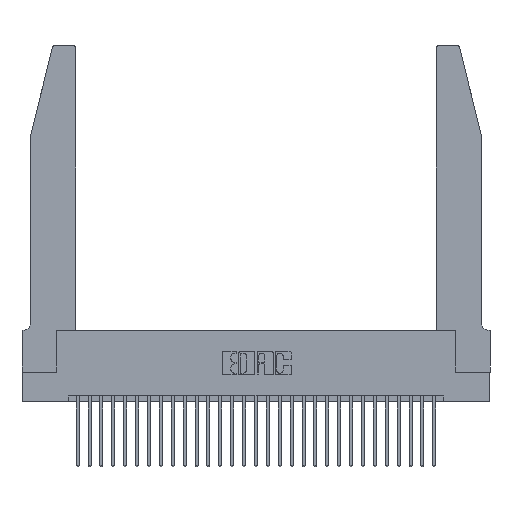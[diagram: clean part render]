
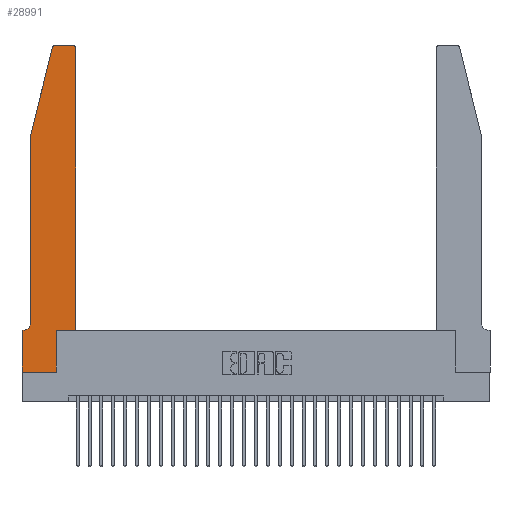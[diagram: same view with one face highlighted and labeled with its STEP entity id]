
A CAD part, top view. The second image highlights one B-rep face of the part: STEP entity #28991.
In plain terms, the highlighted planar face has unit normal (0, 0, 1).
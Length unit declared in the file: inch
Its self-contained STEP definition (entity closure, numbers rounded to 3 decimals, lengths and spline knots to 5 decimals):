
#165 = VECTOR ( 'NONE', #12756, 39.37008 ) ;
#220 = EDGE_CURVE ( 'NONE', #2170, #4722, #12702, .T. ) ;
#1205 = VECTOR ( 'NONE', #4119, 39.37008 ) ;
#1539 = ORIENTED_EDGE ( 'NONE', *, *, #20435, .T. ) ;
#1546 = LINE ( 'NONE', #21854, #14168 ) ;
#1667 = ORIENTED_EDGE ( 'NONE', *, *, #12171, .T. ) ;
#2170 = VERTEX_POINT ( 'NONE', #16006 ) ;
#2358 = CARTESIAN_POINT ( 'NONE',  ( 0.0055, 0.42, 0.37 ) ) ;
#3469 = EDGE_LOOP ( 'NONE', ( #22981, #5084, #25756, #27916, #11546, #19803, #18902, #1539, #1667, #20154, #10247, #19961 ) ) ;
#3696 = CARTESIAN_POINT ( 'NONE',  ( 0.4505, 0.35, 0.37 ) ) ;
#3702 = CARTESIAN_POINT ( 'NONE',  ( 0.4205, 2.72, 0.37 ) ) ;
#3861 = VERTEX_POINT ( 'NONE', #10319 ) ;
#4119 = DIRECTION ( 'NONE',  ( 0., -1., 0. ) ) ;
#4722 = VERTEX_POINT ( 'NONE', #16071 ) ;
#4742 = DIRECTION ( 'NONE',  ( -1., 0., 0. ) ) ;
#5084 = ORIENTED_EDGE ( 'NONE', *, *, #29666, .T. ) ;
#5510 = DIRECTION ( 'NONE',  ( -0.239, -0.971, 0. ) ) ;
#6071 = DIRECTION ( 'NONE',  ( 0., 1., 0. ) ) ;
#6081 = DIRECTION ( 'NONE',  ( 1., 0., 0. ) ) ;
#6169 = CARTESIAN_POINT ( 'NONE',  ( 0.25487, 2.72718, 0.37 ) ) ;
#6411 = VECTOR ( 'NONE', #6950, 39.37008 ) ;
#6533 = LINE ( 'NONE', #10378, #165 ) ;
#6630 = VECTOR ( 'NONE', #6666, 39.37008 ) ;
#6666 = DIRECTION ( 'NONE',  ( 0., -1., 0. ) ) ;
#6726 = EDGE_CURVE ( 'NONE', #9099, #27608, #6533, .T. ) ;
#6950 = DIRECTION ( 'NONE',  ( 1., 0., 0. ) ) ;
#7416 = EDGE_CURVE ( 'NONE', #28107, #9787, #12413, .T. ) ;
#7715 = DIRECTION ( 'NONE',  ( -1., 0., 0. ) ) ;
#7949 = DIRECTION ( 'NONE',  ( 1., 0., 0. ) ) ;
#8011 = CARTESIAN_POINT ( 'NONE',  ( 0.284, 2.72, 0.37 ) ) ;
#8129 = AXIS2_PLACEMENT_3D ( 'NONE', #3702, #20229, #6081 ) ;
#8808 = CARTESIAN_POINT ( 'NONE',  ( 0., 0., 0.37 ) ) ;
#8992 = AXIS2_PLACEMENT_3D ( 'NONE', #8011, #24531, #10399 ) ;
#9099 = VERTEX_POINT ( 'NONE', #26008 ) ;
#9361 = VERTEX_POINT ( 'NONE', #6169 ) ;
#9787 = VERTEX_POINT ( 'NONE', #26584 ) ;
#10247 = ORIENTED_EDGE ( 'NONE', *, *, #17869, .T. ) ;
#10319 = CARTESIAN_POINT ( 'NONE',  ( 0.2865, 0., 0.37 ) ) ;
#10378 = CARTESIAN_POINT ( 'NONE',  ( 0.0755, 0.35, 0.37 ) ) ;
#10399 = DIRECTION ( 'NONE',  ( 1., 0., 0. ) ) ;
#10727 = CIRCLE ( 'NONE', #8992, 0.03 ) ;
#11093 = DIRECTION ( 'NONE',  ( 1., 0., 0. ) ) ;
#11546 = ORIENTED_EDGE ( 'NONE', *, *, #25766, .T. ) ;
#12171 = EDGE_CURVE ( 'NONE', #3861, #2170, #27628, .T. ) ;
#12313 = CARTESIAN_POINT ( 'NONE',  ( 0.2865, 0.35, 0.37 ) ) ;
#12413 = CIRCLE ( 'NONE', #8129, 0.03 ) ;
#12702 = LINE ( 'NONE', #28288, #6411 ) ;
#12756 = DIRECTION ( 'NONE',  ( -1., 0., 0. ) ) ;
#13671 = CARTESIAN_POINT ( 'NONE',  ( 0.0755, 2., 0.37 ) ) ;
#14168 = VECTOR ( 'NONE', #7715, 39.37008 ) ;
#14942 = AXIS2_PLACEMENT_3D ( 'NONE', #19725, #22085, #7949 ) ;
#15823 = CIRCLE ( 'NONE', #25525, 0.07 ) ;
#16006 = CARTESIAN_POINT ( 'NONE',  ( 0.2865, 0.35, 0.37 ) ) ;
#16071 = CARTESIAN_POINT ( 'NONE',  ( 0.4505, 0.35, 0.37 ) ) ;
#16453 = CARTESIAN_POINT ( 'NONE',  ( 0., 0.35, 0.37 ) ) ;
#17087 = DIRECTION ( 'NONE',  ( 0., 1., 0. ) ) ;
#17370 = PLANE ( 'NONE',  #14942 ) ;
#17582 = VECTOR ( 'NONE', #11093, 39.37008 ) ;
#17869 = EDGE_CURVE ( 'NONE', #4722, #28107, #18270, .T. ) ;
#18168 = FACE_OUTER_BOUND ( 'NONE', #3469, .T. ) ;
#18266 = EDGE_CURVE ( 'NONE', #9787, #28975, #1546, .T. ) ;
#18270 = LINE ( 'NONE', #3696, #23809 ) ;
#18298 = CARTESIAN_POINT ( 'NONE',  ( 0., 0., 0.37 ) ) ;
#18902 = ORIENTED_EDGE ( 'NONE', *, *, #21084, .T. ) ;
#18944 = DIRECTION ( 'NONE',  ( 0., 0., -1. ) ) ;
#19310 = VERTEX_POINT ( 'NONE', #30505 ) ;
#19388 = LINE ( 'NONE', #18298, #1205 ) ;
#19636 = CARTESIAN_POINT ( 'NONE',  ( 0.284, 2.75, 0.37 ) ) ;
#19725 = CARTESIAN_POINT ( 'NONE',  ( 0., 0.35, 0.37 ) ) ;
#19803 = ORIENTED_EDGE ( 'NONE', *, *, #6726, .T. ) ;
#19961 = ORIENTED_EDGE ( 'NONE', *, *, #7416, .T. ) ;
#20154 = ORIENTED_EDGE ( 'NONE', *, *, #220, .T. ) ;
#20229 = DIRECTION ( 'NONE',  ( 0., 0., 1. ) ) ;
#20358 = CARTESIAN_POINT ( 'NONE',  ( 0.0755, 0.42, 0.37 ) ) ;
#20435 = EDGE_CURVE ( 'NONE', #25732, #3861, #24577, .T. ) ;
#21084 = EDGE_CURVE ( 'NONE', #27608, #25732, #19388, .T. ) ;
#21854 = CARTESIAN_POINT ( 'NONE',  ( 0.2605, 2.75, 0.37 ) ) ;
#22085 = DIRECTION ( 'NONE',  ( 0., 0., 1. ) ) ;
#22606 = VECTOR ( 'NONE', #5510, 39.37008 ) ;
#22981 = ORIENTED_EDGE ( 'NONE', *, *, #18266, .T. ) ;
#23377 = LINE ( 'NONE', #26657, #22606 ) ;
#23461 = CARTESIAN_POINT ( 'NONE',  ( 0., 0., 0.37 ) ) ;
#23809 = VECTOR ( 'NONE', #6071, 39.37008 ) ;
#24531 = DIRECTION ( 'NONE',  ( 0., 0., 1. ) ) ;
#24577 = LINE ( 'NONE', #8808, #17582 ) ;
#25454 = LINE ( 'NONE', #13671, #6630 ) ;
#25525 = AXIS2_PLACEMENT_3D ( 'NONE', #2358, #18944, #4742 ) ;
#25732 = VERTEX_POINT ( 'NONE', #23461 ) ;
#25756 = ORIENTED_EDGE ( 'NONE', *, *, #28367, .T. ) ;
#25766 = EDGE_CURVE ( 'NONE', #27359, #9099, #15823, .T. ) ;
#26008 = CARTESIAN_POINT ( 'NONE',  ( 0.0055, 0.35, 0.37 ) ) ;
#26584 = CARTESIAN_POINT ( 'NONE',  ( 0.4205, 2.75, 0.37 ) ) ;
#26657 = CARTESIAN_POINT ( 'NONE',  ( 0.0755, 2., 0.37 ) ) ;
#26904 = VECTOR ( 'NONE', #17087, 39.37008 ) ;
#27359 = VERTEX_POINT ( 'NONE', #20358 ) ;
#27608 = VERTEX_POINT ( 'NONE', #16453 ) ;
#27628 = LINE ( 'NONE', #12313, #26904 ) ;
#27916 = ORIENTED_EDGE ( 'NONE', *, *, #30030, .T. ) ;
#28107 = VERTEX_POINT ( 'NONE', #28220 ) ;
#28220 = CARTESIAN_POINT ( 'NONE',  ( 0.4505, 2.72, 0.37 ) ) ;
#28288 = CARTESIAN_POINT ( 'NONE',  ( 0.4505, 0.35, 0.37 ) ) ;
#28367 = EDGE_CURVE ( 'NONE', #9361, #19310, #23377, .T. ) ;
#28975 = VERTEX_POINT ( 'NONE', #19636 ) ;
#28991 = ADVANCED_FACE ( 'NONE', ( #18168 ), #17370, .T. ) ;
#29666 = EDGE_CURVE ( 'NONE', #28975, #9361, #10727, .T. ) ;
#30030 = EDGE_CURVE ( 'NONE', #19310, #27359, #25454, .T. ) ;
#30505 = CARTESIAN_POINT ( 'NONE',  ( 0.0755, 2., 0.37 ) ) ;
